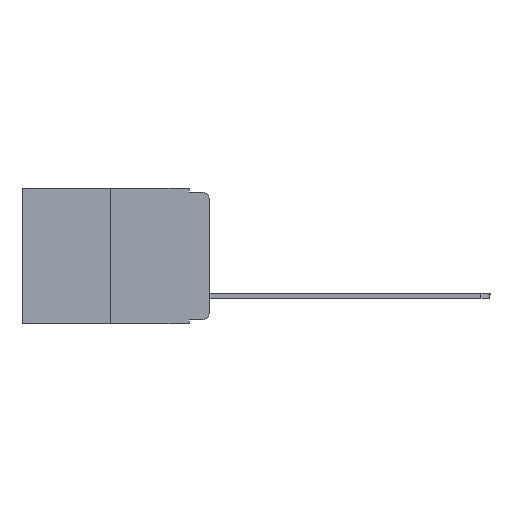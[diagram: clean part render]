
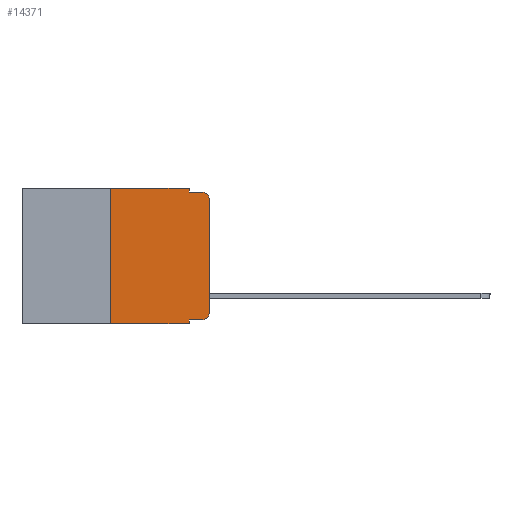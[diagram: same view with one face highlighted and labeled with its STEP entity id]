
A CAD part, left-side view. The second image highlights one B-rep face of the part: STEP entity #14371.
In plain terms, the highlighted planar face has unit normal (-1, 0, 0).
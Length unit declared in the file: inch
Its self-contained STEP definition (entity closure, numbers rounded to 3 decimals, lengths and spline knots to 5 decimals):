
#43 = CIRCLE ( 'NONE', #5789, 0.02 ) ;
#314 = EDGE_CURVE ( 'NONE', #4123, #7409, #3327, .T. ) ;
#427 = AXIS2_PLACEMENT_3D ( 'NONE', #5990, #16306, #12471 ) ;
#456 = CARTESIAN_POINT ( 'NONE',  ( 0., 0.051, -0.333 ) ) ;
#638 = CARTESIAN_POINT ( 'NONE',  ( 0., 0.051, 0. ) ) ;
#1309 = ORIENTED_EDGE ( 'NONE', *, *, #9011, .F. ) ;
#1397 = CARTESIAN_POINT ( 'NONE',  ( 0., 0., -0.313 ) ) ;
#1442 = EDGE_CURVE ( 'NONE', #7409, #8929, #14539, .T. ) ;
#1493 = ORIENTED_EDGE ( 'NONE', *, *, #14184, .T. ) ;
#1579 = CARTESIAN_POINT ( 'NONE',  ( 0., 0.051, -0.343 ) ) ;
#1712 = VECTOR ( 'NONE', #11822, 39.37008 ) ;
#1977 = CARTESIAN_POINT ( 'NONE',  ( 0., 0.02, -0.01 ) ) ;
#2329 = EDGE_CURVE ( 'NONE', #11540, #13023, #7041, .T. ) ;
#2414 = CARTESIAN_POINT ( 'NONE',  ( 0., 0.02, -0.333 ) ) ;
#2428 = DIRECTION ( 'NONE',  ( -1., 0., 0. ) ) ;
#2654 = EDGE_CURVE ( 'NONE', #6869, #13023, #9240, .T. ) ;
#2764 = DIRECTION ( 'NONE',  ( 0., -1., 0. ) ) ;
#2897 = CARTESIAN_POINT ( 'NONE',  ( 0., 0.02, -0.313 ) ) ;
#2951 = VERTEX_POINT ( 'NONE', #2414 ) ;
#3089 = CARTESIAN_POINT ( 'NONE',  ( 0., 0., 0. ) ) ;
#3201 = DIRECTION ( 'NONE',  ( 0., 0., -1. ) ) ;
#3327 = LINE ( 'NONE', #12689, #10360 ) ;
#3545 = CARTESIAN_POINT ( 'NONE',  ( 0., 0.02, -0.03 ) ) ;
#3700 = CARTESIAN_POINT ( 'NONE',  ( 0., 0.25, 0. ) ) ;
#4123 = VERTEX_POINT ( 'NONE', #638 ) ;
#4162 = CARTESIAN_POINT ( 'NONE',  ( 0., 0.473, 0. ) ) ;
#4477 = CARTESIAN_POINT ( 'NONE',  ( 0., 0.051, 0. ) ) ;
#4673 = CARTESIAN_POINT ( 'NONE',  ( 0., 0.25, -0.343 ) ) ;
#5529 = LINE ( 'NONE', #14600, #9603 ) ;
#5652 = ORIENTED_EDGE ( 'NONE', *, *, #8904, .T. ) ;
#5789 = AXIS2_PLACEMENT_3D ( 'NONE', #2897, #8182, #13473 ) ;
#5990 = CARTESIAN_POINT ( 'NONE',  ( 0., 0.473, 0. ) ) ;
#6101 = VERTEX_POINT ( 'NONE', #1397 ) ;
#6171 = AXIS2_PLACEMENT_3D ( 'NONE', #3545, #2428, #8743 ) ;
#6695 = CARTESIAN_POINT ( 'NONE',  ( 0., 0.051, -0.333 ) ) ;
#6869 = VERTEX_POINT ( 'NONE', #4673 ) ;
#7041 = LINE ( 'NONE', #4477, #11673 ) ;
#7409 = VERTEX_POINT ( 'NONE', #12833 ) ;
#7747 = DIRECTION ( 'NONE',  ( 0., -1., 0. ) ) ;
#7955 = FACE_OUTER_BOUND ( 'NONE', #9973, .T. ) ;
#8182 = DIRECTION ( 'NONE',  ( -1., 0., 0. ) ) ;
#8537 = EDGE_CURVE ( 'NONE', #6101, #11326, #14468, .T. ) ;
#8549 = PLANE ( 'NONE',  #427 ) ;
#8650 = ORIENTED_EDGE ( 'NONE', *, *, #8537, .T. ) ;
#8743 = DIRECTION ( 'NONE',  ( 0., 0., -1. ) ) ;
#8863 = DIRECTION ( 'NONE',  ( 0., 0., -1. ) ) ;
#8904 = EDGE_CURVE ( 'NONE', #2951, #6101, #43, .T. ) ;
#8929 = VERTEX_POINT ( 'NONE', #1977 ) ;
#9011 = EDGE_CURVE ( 'NONE', #6869, #14159, #5529, .T. ) ;
#9240 = LINE ( 'NONE', #14448, #12112 ) ;
#9379 = ORIENTED_EDGE ( 'NONE', *, *, #2654, .T. ) ;
#9603 = VECTOR ( 'NONE', #13649, 39.37008 ) ;
#9973 = EDGE_LOOP ( 'NONE', ( #8650, #1493, #13813, #16017, #10983, #1309, #9379, #14660, #15068, #5652 ) ) ;
#10245 = VECTOR ( 'NONE', #7747, 39.37008 ) ;
#10360 = VECTOR ( 'NONE', #8863, 39.37008 ) ;
#10438 = EDGE_CURVE ( 'NONE', #14159, #4123, #11680, .T. ) ;
#10478 = DIRECTION ( 'NONE',  ( 0., -1., 0. ) ) ;
#10510 = CARTESIAN_POINT ( 'NONE',  ( 0., 0.051, -0.01 ) ) ;
#10983 = ORIENTED_EDGE ( 'NONE', *, *, #10438, .F. ) ;
#11326 = VERTEX_POINT ( 'NONE', #12903 ) ;
#11540 = VERTEX_POINT ( 'NONE', #6695 ) ;
#11627 = DIRECTION ( 'NONE',  ( 0., -1., 0. ) ) ;
#11673 = VECTOR ( 'NONE', #3201, 39.37008 ) ;
#11680 = LINE ( 'NONE', #4162, #16178 ) ;
#11822 = DIRECTION ( 'NONE',  ( 0., 0., 1. ) ) ;
#12112 = VECTOR ( 'NONE', #2764, 39.37008 ) ;
#12146 = LINE ( 'NONE', #456, #10245 ) ;
#12471 = DIRECTION ( 'NONE',  ( 0., 0., -1. ) ) ;
#12689 = CARTESIAN_POINT ( 'NONE',  ( 0., 0.051, 0. ) ) ;
#12833 = CARTESIAN_POINT ( 'NONE',  ( 0., 0.051, -0.01 ) ) ;
#12903 = CARTESIAN_POINT ( 'NONE',  ( 0., 0., -0.03 ) ) ;
#13023 = VERTEX_POINT ( 'NONE', #1579 ) ;
#13473 = DIRECTION ( 'NONE',  ( 0., 0., -1. ) ) ;
#13649 = DIRECTION ( 'NONE',  ( 0., 0., 1. ) ) ;
#13813 = ORIENTED_EDGE ( 'NONE', *, *, #1442, .F. ) ;
#13953 = EDGE_CURVE ( 'NONE', #11540, #2951, #12146, .T. ) ;
#14082 = CIRCLE ( 'NONE', #6171, 0.02 ) ;
#14159 = VERTEX_POINT ( 'NONE', #3700 ) ;
#14184 = EDGE_CURVE ( 'NONE', #11326, #8929, #14082, .T. ) ;
#14371 = ADVANCED_FACE ( 'NONE', ( #7955 ), #8549, .F. ) ;
#14448 = CARTESIAN_POINT ( 'NONE',  ( 0., 0.473, -0.343 ) ) ;
#14468 = LINE ( 'NONE', #3089, #1712 ) ;
#14539 = LINE ( 'NONE', #10510, #15625 ) ;
#14600 = CARTESIAN_POINT ( 'NONE',  ( 0., 0.25, 0. ) ) ;
#14660 = ORIENTED_EDGE ( 'NONE', *, *, #2329, .F. ) ;
#15068 = ORIENTED_EDGE ( 'NONE', *, *, #13953, .T. ) ;
#15625 = VECTOR ( 'NONE', #11627, 39.37008 ) ;
#16017 = ORIENTED_EDGE ( 'NONE', *, *, #314, .F. ) ;
#16178 = VECTOR ( 'NONE', #10478, 39.37008 ) ;
#16306 = DIRECTION ( 'NONE',  ( 1., 0., 0. ) ) ;
